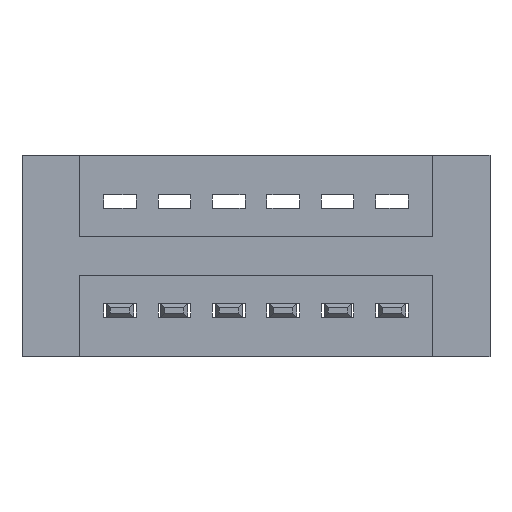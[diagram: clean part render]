
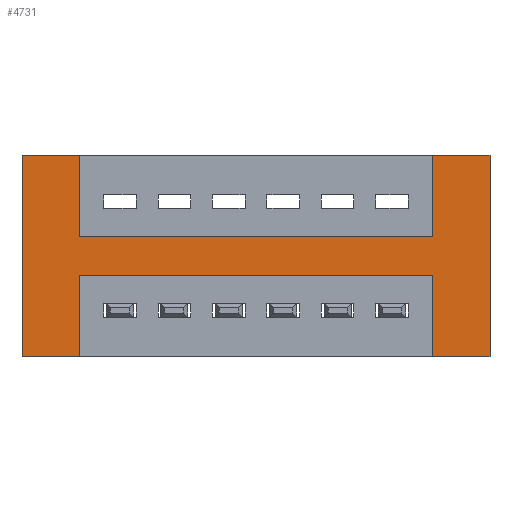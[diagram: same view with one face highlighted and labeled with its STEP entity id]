
A CAD part, front view. The second image highlights one B-rep face of the part: STEP entity #4731.
In plain terms, the highlighted planar face has unit normal (0, -1, 0).
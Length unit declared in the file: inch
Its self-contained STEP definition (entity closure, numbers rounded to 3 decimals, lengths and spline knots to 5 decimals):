
#239 = CARTESIAN_POINT ( 'NONE',  ( 1.1475, 0., 0. ) ) ;
#265 = CARTESIAN_POINT ( 'NONE',  ( 0.3925, 0., -0.22 ) ) ;
#430 = ORIENTED_EDGE ( 'NONE', *, *, #1910, .F. ) ;
#446 = LINE ( 'NONE', #6032, #7700 ) ;
#579 = EDGE_CURVE ( 'NONE', #6085, #5765, #3559, .T. ) ;
#659 = ORIENTED_EDGE ( 'NONE', *, *, #1149, .F. ) ;
#698 = VECTOR ( 'NONE', #851, 39.37008 ) ;
#813 = AXIS2_PLACEMENT_3D ( 'NONE', #7020, #6354, #6388 ) ;
#851 = DIRECTION ( 'NONE',  ( 1., 0., 0. ) ) ;
#1149 = EDGE_CURVE ( 'NONE', #7189, #7656, #5207, .T. ) ;
#1165 = EDGE_CURVE ( 'NONE', #2599, #5231, #5423, .T. ) ;
#1170 = LINE ( 'NONE', #2981, #6573 ) ;
#1476 = CARTESIAN_POINT ( 'NONE',  ( 0.3925, 0., -0.15 ) ) ;
#1504 = DIRECTION ( 'NONE',  ( 0., 0., -1. ) ) ;
#1537 = ORIENTED_EDGE ( 'NONE', *, *, #6691, .F. ) ;
#1539 = LINE ( 'NONE', #8902, #5120 ) ;
#1594 = VERTEX_POINT ( 'NONE', #1476 ) ;
#1656 = DIRECTION ( 'NONE',  ( 1., 0., 0. ) ) ;
#1658 = ORIENTED_EDGE ( 'NONE', *, *, #579, .F. ) ;
#1910 = EDGE_CURVE ( 'NONE', #6094, #5044, #446, .T. ) ;
#2063 = VERTEX_POINT ( 'NONE', #7702 ) ;
#2196 = VERTEX_POINT ( 'NONE', #7933 ) ;
#2207 = CARTESIAN_POINT ( 'NONE',  ( 0., 0., -0.37 ) ) ;
#2282 = VECTOR ( 'NONE', #1656, 39.37008 ) ;
#2287 = LINE ( 'NONE', #5002, #5806 ) ;
#2364 = CARTESIAN_POINT ( 'NONE',  ( 0., 0., -0.37 ) ) ;
#2467 = DIRECTION ( 'NONE',  ( 0., 0., 1. ) ) ;
#2575 = CARTESIAN_POINT ( 'NONE',  ( 1.0425, 0., -0.37 ) ) ;
#2599 = VERTEX_POINT ( 'NONE', #4654 ) ;
#2704 = DIRECTION ( 'NONE',  ( -1., 0., 0. ) ) ;
#2762 = DIRECTION ( 'NONE',  ( -1., 0., 0. ) ) ;
#2959 = ORIENTED_EDGE ( 'NONE', *, *, #8683, .F. ) ;
#2981 = CARTESIAN_POINT ( 'NONE',  ( 0.3925, 0., -0.37 ) ) ;
#3028 = VECTOR ( 'NONE', #2467, 39.37008 ) ;
#3149 = ORIENTED_EDGE ( 'NONE', *, *, #8063, .F. ) ;
#3251 = EDGE_CURVE ( 'NONE', #5044, #6868, #8066, .T. ) ;
#3327 = VECTOR ( 'NONE', #2704, 39.37008 ) ;
#3414 = ORIENTED_EDGE ( 'NONE', *, *, #7802, .T. ) ;
#3512 = CARTESIAN_POINT ( 'NONE',  ( 1.1475, 0., -0.37 ) ) ;
#3549 = VECTOR ( 'NONE', #2762, 39.37008 ) ;
#3559 = LINE ( 'NONE', #4204, #6927 ) ;
#3587 = LINE ( 'NONE', #8072, #8569 ) ;
#3835 = DIRECTION ( 'NONE',  ( 1., 0., 0. ) ) ;
#4103 = EDGE_CURVE ( 'NONE', #2196, #2063, #7662, .T. ) ;
#4181 = ORIENTED_EDGE ( 'NONE', *, *, #1165, .F. ) ;
#4204 = CARTESIAN_POINT ( 'NONE',  ( 0.3925, 0., -0.22 ) ) ;
#4284 = FACE_OUTER_BOUND ( 'NONE', #4723, .T. ) ;
#4413 = DIRECTION ( 'NONE',  ( -1., 0., 0. ) ) ;
#4654 = CARTESIAN_POINT ( 'NONE',  ( 0.3925, 0., -0.37 ) ) ;
#4723 = EDGE_LOOP ( 'NONE', ( #5294, #8783, #430, #3149, #1537, #5186, #3414, #4181, #4946, #1658, #2959, #659 ) ) ;
#4731 = ADVANCED_FACE ( 'NONE', ( #4284 ), #5826, .T. ) ;
#4946 = ORIENTED_EDGE ( 'NONE', *, *, #7349, .F. ) ;
#4984 = CARTESIAN_POINT ( 'NONE',  ( 0., 0., 0. ) ) ;
#5002 = CARTESIAN_POINT ( 'NONE',  ( 0.3925, 0., 0. ) ) ;
#5044 = VERTEX_POINT ( 'NONE', #7674 ) ;
#5101 = EDGE_CURVE ( 'NONE', #7189, #6868, #6854, .T. ) ;
#5120 = VECTOR ( 'NONE', #3835, 39.37008 ) ;
#5186 = ORIENTED_EDGE ( 'NONE', *, *, #4103, .F. ) ;
#5207 = LINE ( 'NONE', #2364, #3327 ) ;
#5231 = VERTEX_POINT ( 'NONE', #5609 ) ;
#5294 = ORIENTED_EDGE ( 'NONE', *, *, #5101, .T. ) ;
#5423 = LINE ( 'NONE', #2207, #3549 ) ;
#5609 = CARTESIAN_POINT ( 'NONE',  ( 0.2875, 0., -0.37 ) ) ;
#5765 = VERTEX_POINT ( 'NONE', #265 ) ;
#5806 = VECTOR ( 'NONE', #8182, 39.37008 ) ;
#5826 = PLANE ( 'NONE',  #813 ) ;
#6032 = CARTESIAN_POINT ( 'NONE',  ( 1.0425, 0., 0. ) ) ;
#6085 = VERTEX_POINT ( 'NONE', #7027 ) ;
#6094 = VERTEX_POINT ( 'NONE', #7967 ) ;
#6354 = DIRECTION ( 'NONE',  ( 0., -1., 0. ) ) ;
#6388 = DIRECTION ( 'NONE',  ( 0., 0., -1. ) ) ;
#6573 = VECTOR ( 'NONE', #1504, 39.37008 ) ;
#6587 = CARTESIAN_POINT ( 'NONE',  ( 1.0425, 0., -0.37 ) ) ;
#6691 = EDGE_CURVE ( 'NONE', #2063, #1594, #2287, .T. ) ;
#6854 = LINE ( 'NONE', #239, #7742 ) ;
#6868 = VERTEX_POINT ( 'NONE', #7769 ) ;
#6876 = DIRECTION ( 'NONE',  ( 0., 0., 1. ) ) ;
#6927 = VECTOR ( 'NONE', #4413, 39.37008 ) ;
#7020 = CARTESIAN_POINT ( 'NONE',  ( 0., 0., -0.37 ) ) ;
#7027 = CARTESIAN_POINT ( 'NONE',  ( 1.0425, 0., -0.22 ) ) ;
#7189 = VERTEX_POINT ( 'NONE', #3512 ) ;
#7349 = EDGE_CURVE ( 'NONE', #5765, #2599, #1170, .T. ) ;
#7563 = DIRECTION ( 'NONE',  ( 0., 0., 1. ) ) ;
#7656 = VERTEX_POINT ( 'NONE', #2575 ) ;
#7662 = LINE ( 'NONE', #4984, #2282 ) ;
#7674 = CARTESIAN_POINT ( 'NONE',  ( 1.0425, 0., 0. ) ) ;
#7700 = VECTOR ( 'NONE', #7563, 39.37008 ) ;
#7702 = CARTESIAN_POINT ( 'NONE',  ( 0.3925, 0., 0. ) ) ;
#7742 = VECTOR ( 'NONE', #6876, 39.37008 ) ;
#7769 = CARTESIAN_POINT ( 'NONE',  ( 1.1475, 0., 0. ) ) ;
#7802 = EDGE_CURVE ( 'NONE', #2196, #5231, #3587, .T. ) ;
#7933 = CARTESIAN_POINT ( 'NONE',  ( 0.2875, 0., 0. ) ) ;
#7967 = CARTESIAN_POINT ( 'NONE',  ( 1.0425, 0., -0.15 ) ) ;
#8063 = EDGE_CURVE ( 'NONE', #1594, #6094, #1539, .T. ) ;
#8066 = LINE ( 'NONE', #8714, #698 ) ;
#8072 = CARTESIAN_POINT ( 'NONE',  ( 0.2875, 0., 0. ) ) ;
#8117 = LINE ( 'NONE', #6587, #3028 ) ;
#8182 = DIRECTION ( 'NONE',  ( 0., 0., -1. ) ) ;
#8569 = VECTOR ( 'NONE', #8628, 39.37008 ) ;
#8628 = DIRECTION ( 'NONE',  ( 0., 0., -1. ) ) ;
#8683 = EDGE_CURVE ( 'NONE', #7656, #6085, #8117, .T. ) ;
#8714 = CARTESIAN_POINT ( 'NONE',  ( 0., 0., 0. ) ) ;
#8783 = ORIENTED_EDGE ( 'NONE', *, *, #3251, .F. ) ;
#8902 = CARTESIAN_POINT ( 'NONE',  ( 0.3925, 0., -0.15 ) ) ;
